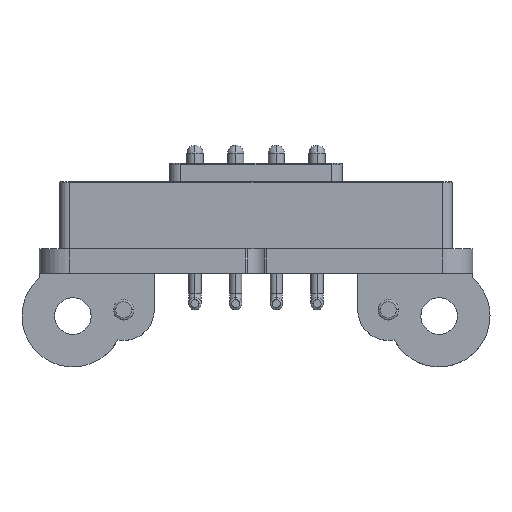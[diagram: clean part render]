
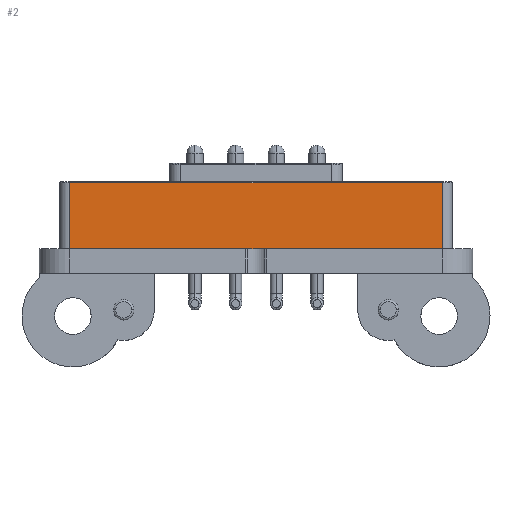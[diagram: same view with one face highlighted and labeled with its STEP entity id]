
A CAD part, top view. The second image highlights one B-rep face of the part: STEP entity #2.
In plain terms, the highlighted planar face has unit normal (0, 0, 1).
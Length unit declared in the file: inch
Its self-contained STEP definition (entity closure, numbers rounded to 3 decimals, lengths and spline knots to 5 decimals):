
#2 = ADVANCED_FACE ( 'NONE', ( #10213 ), #1705, .F. ) ;
#248 = ORIENTED_EDGE ( 'NONE', *, *, #7628, .T. ) ;
#437 = EDGE_CURVE ( 'NONE', #8165, #5715, #4218, .T. ) ;
#608 = AXIS2_PLACEMENT_3D ( 'NONE', #8551, #6745, #9221 ) ;
#687 = LINE ( 'NONE', #5699, #6026 ) ;
#829 = CARTESIAN_POINT ( 'NONE',  ( -0.36024, 0.04724, 0.08071 ) ) ;
#1266 = ORIENTED_EDGE ( 'NONE', *, *, #4449, .T. ) ;
#1498 = LINE ( 'NONE', #6429, #5716 ) ;
#1702 = VERTEX_POINT ( 'NONE', #7838 ) ;
#1705 = PLANE ( 'NONE',  #608 ) ;
#2082 = VERTEX_POINT ( 'NONE', #7638 ) ;
#2318 = CARTESIAN_POINT ( 'NONE',  ( -0.37992, 0.04724, 0.08071 ) ) ;
#3203 = DIRECTION ( 'NONE',  ( -1., 0., 0. ) ) ;
#3320 = ORIENTED_EDGE ( 'NONE', *, *, #9492, .T. ) ;
#4136 = DIRECTION ( 'NONE',  ( 0., 1., 0. ) ) ;
#4218 = LINE ( 'NONE', #2318, #5286 ) ;
#4449 = EDGE_CURVE ( 'NONE', #1702, #8165, #10021, .T. ) ;
#4865 = CARTESIAN_POINT ( 'NONE',  ( 0.36024, 0.04724, 0.08071 ) ) ;
#5105 = CARTESIAN_POINT ( 'NONE',  ( -0.36024, 0.17717, 0.08071 ) ) ;
#5286 = VECTOR ( 'NONE', #5723, 39.37008 ) ;
#5699 = CARTESIAN_POINT ( 'NONE',  ( 0.36024, 0.17717, 0.08071 ) ) ;
#5715 = VERTEX_POINT ( 'NONE', #4865 ) ;
#5716 = VECTOR ( 'NONE', #3203, 39.37008 ) ;
#5723 = DIRECTION ( 'NONE',  ( 1., 0., 0. ) ) ;
#6026 = VECTOR ( 'NONE', #4136, 39.37008 ) ;
#6429 = CARTESIAN_POINT ( 'NONE',  ( -0.37992, 0.1752, 0.08071 ) ) ;
#6682 = ORIENTED_EDGE ( 'NONE', *, *, #437, .T. ) ;
#6745 = DIRECTION ( 'NONE',  ( 0., 0., -1. ) ) ;
#7628 = EDGE_CURVE ( 'NONE', #5715, #2082, #687, .T. ) ;
#7638 = CARTESIAN_POINT ( 'NONE',  ( 0.36024, 0.1752, 0.08071 ) ) ;
#7838 = CARTESIAN_POINT ( 'NONE',  ( -0.36024, 0.1752, 0.08071 ) ) ;
#8165 = VERTEX_POINT ( 'NONE', #829 ) ;
#8551 = CARTESIAN_POINT ( 'NONE',  ( -0.37992, 0.17717, 0.08071 ) ) ;
#9221 = DIRECTION ( 'NONE',  ( -1., 0., 0. ) ) ;
#9492 = EDGE_CURVE ( 'NONE', #2082, #1702, #1498, .T. ) ;
#10021 = LINE ( 'NONE', #5105, #10326 ) ;
#10178 = DIRECTION ( 'NONE',  ( 0., -1., 0. ) ) ;
#10213 = FACE_OUTER_BOUND ( 'NONE', #10680, .T. ) ;
#10326 = VECTOR ( 'NONE', #10178, 39.37008 ) ;
#10680 = EDGE_LOOP ( 'NONE', ( #248, #3320, #1266, #6682 ) ) ;
